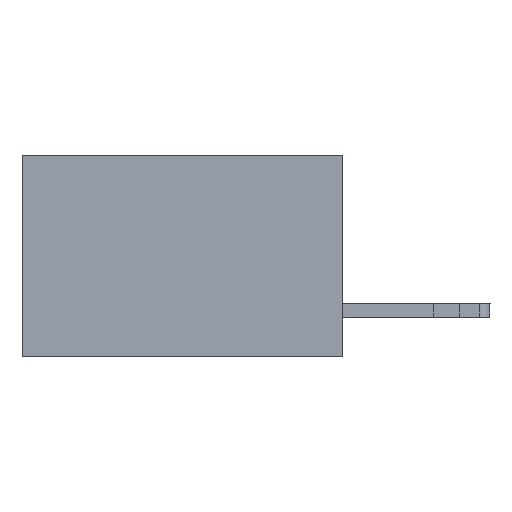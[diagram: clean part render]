
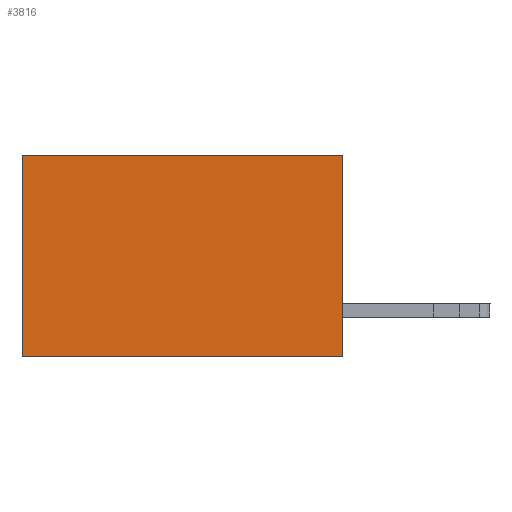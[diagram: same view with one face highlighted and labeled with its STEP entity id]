
A CAD part, left-side view. The second image highlights one B-rep face of the part: STEP entity #3816.
In plain terms, the highlighted planar face has unit normal (-1, 0, 0).
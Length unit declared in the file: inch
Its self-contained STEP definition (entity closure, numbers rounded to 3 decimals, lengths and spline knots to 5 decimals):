
#308 = CARTESIAN_POINT ( 'NONE',  ( 0.277, 0., -0.37 ) ) ;
#505 = DIRECTION ( 'NONE',  ( 1., 0., 0. ) ) ;
#566 = VERTEX_POINT ( 'NONE', #3721 ) ;
#976 = DIRECTION ( 'NONE',  ( 0., 0., -1. ) ) ;
#1043 = PLANE ( 'NONE',  #8405 ) ;
#1163 = LINE ( 'NONE', #11787, #17053 ) ;
#1186 = FACE_OUTER_BOUND ( 'NONE', #18980, .T. ) ;
#2245 = VERTEX_POINT ( 'NONE', #9611 ) ;
#2253 = CARTESIAN_POINT ( 'NONE',  ( 0.277, 0., -0.37 ) ) ;
#2333 = EDGE_CURVE ( 'NONE', #3583, #2389, #8527, .T. ) ;
#2389 = VERTEX_POINT ( 'NONE', #14852 ) ;
#3583 = VERTEX_POINT ( 'NONE', #10203 ) ;
#3721 = CARTESIAN_POINT ( 'NONE',  ( 0.277, 0., 0. ) ) ;
#3816 = ADVANCED_FACE ( 'NONE', ( #1186 ), #1043, .F. ) ;
#4271 = EDGE_CURVE ( 'NONE', #566, #2245, #1163, .T. ) ;
#4429 = VECTOR ( 'NONE', #17064, 39.37008 ) ;
#7262 = ORIENTED_EDGE ( 'NONE', *, *, #2333, .F. ) ;
#7400 = LINE ( 'NONE', #15324, #19086 ) ;
#7480 = LINE ( 'NONE', #2253, #11588 ) ;
#8405 = AXIS2_PLACEMENT_3D ( 'NONE', #308, #505, #976 ) ;
#8527 = LINE ( 'NONE', #19240, #4429 ) ;
#9611 = CARTESIAN_POINT ( 'NONE',  ( 0.277, 0.59, 0. ) ) ;
#10203 = CARTESIAN_POINT ( 'NONE',  ( 0.277, 0., -0.37 ) ) ;
#10890 = ORIENTED_EDGE ( 'NONE', *, *, #17093, .T. ) ;
#11537 = DIRECTION ( 'NONE',  ( 0., 1., 0. ) ) ;
#11588 = VECTOR ( 'NONE', #13066, 39.37008 ) ;
#11787 = CARTESIAN_POINT ( 'NONE',  ( 0.277, 0., 0. ) ) ;
#12087 = EDGE_CURVE ( 'NONE', #566, #3583, #7480, .T. ) ;
#13066 = DIRECTION ( 'NONE',  ( 0., 0., -1. ) ) ;
#14852 = CARTESIAN_POINT ( 'NONE',  ( 0.277, 0.59, -0.37 ) ) ;
#15324 = CARTESIAN_POINT ( 'NONE',  ( 0.277, 0.59, -0.37 ) ) ;
#16825 = ORIENTED_EDGE ( 'NONE', *, *, #12087, .F. ) ;
#17053 = VECTOR ( 'NONE', #11537, 39.37008 ) ;
#17064 = DIRECTION ( 'NONE',  ( 0., 1., 0. ) ) ;
#17093 = EDGE_CURVE ( 'NONE', #2245, #2389, #7400, .T. ) ;
#17299 = ORIENTED_EDGE ( 'NONE', *, *, #4271, .T. ) ;
#18980 = EDGE_LOOP ( 'NONE', ( #10890, #7262, #16825, #17299 ) ) ;
#19086 = VECTOR ( 'NONE', #19905, 39.37008 ) ;
#19240 = CARTESIAN_POINT ( 'NONE',  ( 0.277, 0., -0.37 ) ) ;
#19905 = DIRECTION ( 'NONE',  ( 0., 0., -1. ) ) ;
